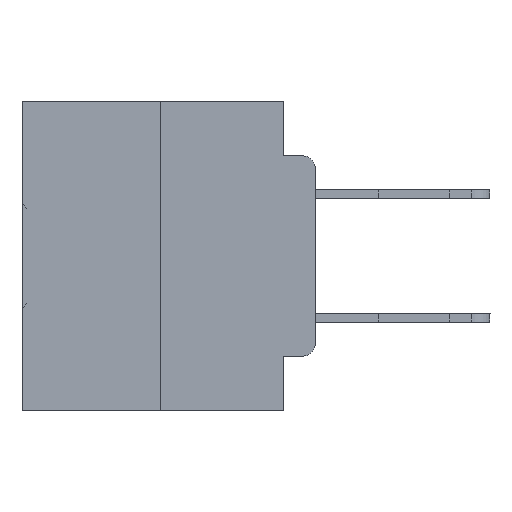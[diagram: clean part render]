
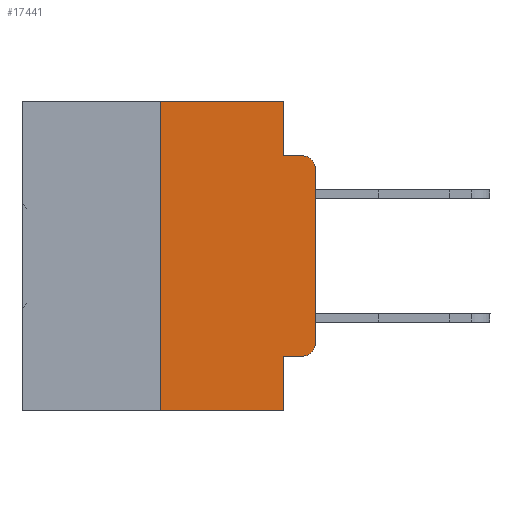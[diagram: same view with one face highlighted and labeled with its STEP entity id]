
A CAD part, left-side view. The second image highlights one B-rep face of the part: STEP entity #17441.
In plain terms, the highlighted planar face has unit normal (-1, 0, 0).
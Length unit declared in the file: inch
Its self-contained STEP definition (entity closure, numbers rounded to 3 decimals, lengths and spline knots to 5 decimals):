
#328 = VECTOR ( 'NONE', #32513, 39.37008 ) ;
#604 = EDGE_CURVE ( 'NONE', #28503, #11090, #23634, .T. ) ;
#620 = ORIENTED_EDGE ( 'NONE', *, *, #7553, .T. ) ;
#666 = CARTESIAN_POINT ( 'NONE',  ( 0., 0.02, -0.0885 ) ) ;
#913 = DIRECTION ( 'NONE',  ( 0., -1., 0. ) ) ;
#926 = CARTESIAN_POINT ( 'NONE',  ( 0., 0.051, -0.0885 ) ) ;
#1120 = EDGE_CURVE ( 'NONE', #25162, #10186, #12783, .T. ) ;
#1220 = DIRECTION ( 'NONE',  ( 0., 0., -1. ) ) ;
#1503 = AXIS2_PLACEMENT_3D ( 'NONE', #24187, #26630, #21522 ) ;
#1647 = DIRECTION ( 'NONE',  ( 0., 0., -1. ) ) ;
#1750 = CARTESIAN_POINT ( 'NONE',  ( 0., 0.25, -0.5 ) ) ;
#1977 = LINE ( 'NONE', #24766, #22276 ) ;
#2507 = DIRECTION ( 'NONE',  ( 0., 0., 1. ) ) ;
#3625 = DIRECTION ( 'NONE',  ( 0., 0., -1. ) ) ;
#4044 = CARTESIAN_POINT ( 'NONE',  ( 0., 0.051, -0.0885 ) ) ;
#5214 = VERTEX_POINT ( 'NONE', #25886 ) ;
#5692 = LINE ( 'NONE', #13133, #20597 ) ;
#6142 = VERTEX_POINT ( 'NONE', #18180 ) ;
#7553 = EDGE_CURVE ( 'NONE', #28503, #25162, #12108, .T. ) ;
#7687 = CARTESIAN_POINT ( 'NONE',  ( 0., 0.051, 0. ) ) ;
#8084 = ORIENTED_EDGE ( 'NONE', *, *, #31767, .T. ) ;
#8592 = ORIENTED_EDGE ( 'NONE', *, *, #604, .F. ) ;
#9708 = ORIENTED_EDGE ( 'NONE', *, *, #27085, .F. ) ;
#9734 = CARTESIAN_POINT ( 'NONE',  ( 0., 0.02, -0.3915 ) ) ;
#10186 = VERTEX_POINT ( 'NONE', #22478 ) ;
#10661 = EDGE_CURVE ( 'NONE', #28291, #11090, #28951, .T. ) ;
#10670 = LINE ( 'NONE', #926, #328 ) ;
#11090 = VERTEX_POINT ( 'NONE', #18429 ) ;
#11204 = CARTESIAN_POINT ( 'NONE',  ( 0., 0.051, -0.4115 ) ) ;
#12108 = LINE ( 'NONE', #24757, #22501 ) ;
#12713 = DIRECTION ( 'NONE',  ( 0., -1., 0. ) ) ;
#12783 = CIRCLE ( 'NONE', #13055, 0.02 ) ;
#12868 = DIRECTION ( 'NONE',  ( 0., 0., -1. ) ) ;
#13055 = AXIS2_PLACEMENT_3D ( 'NONE', #9734, #33575, #1647 ) ;
#13133 = CARTESIAN_POINT ( 'NONE',  ( 0., 0., 0. ) ) ;
#13678 = VECTOR ( 'NONE', #12868, 39.37008 ) ;
#13772 = EDGE_CURVE ( 'NONE', #29614, #30503, #14657, .T. ) ;
#13831 = ORIENTED_EDGE ( 'NONE', *, *, #27044, .F. ) ;
#14417 = VECTOR ( 'NONE', #12713, 39.37008 ) ;
#14657 = LINE ( 'NONE', #24811, #29194 ) ;
#14684 = DIRECTION ( 'NONE',  ( 0., -1., 0. ) ) ;
#15313 = CARTESIAN_POINT ( 'NONE',  ( 0., 0.25, 0. ) ) ;
#16434 = EDGE_CURVE ( 'NONE', #5214, #17668, #28692, .T. ) ;
#16657 = EDGE_CURVE ( 'NONE', #28291, #6142, #30323, .T. ) ;
#17441 = ADVANCED_FACE ( 'NONE', ( #17785 ), #19046, .F. ) ;
#17668 = VERTEX_POINT ( 'NONE', #666 ) ;
#17785 = FACE_OUTER_BOUND ( 'NONE', #25839, .T. ) ;
#18180 = CARTESIAN_POINT ( 'NONE',  ( 0., 0.25, 0. ) ) ;
#18429 = CARTESIAN_POINT ( 'NONE',  ( 0., 0.051, -0.5 ) ) ;
#19046 = PLANE ( 'NONE',  #1503 ) ;
#19600 = CARTESIAN_POINT ( 'NONE',  ( 0., 0.02, -0.1085 ) ) ;
#20140 = CARTESIAN_POINT ( 'NONE',  ( 0., 0.02, -0.4115 ) ) ;
#20597 = VECTOR ( 'NONE', #2507, 39.37008 ) ;
#20775 = ORIENTED_EDGE ( 'NONE', *, *, #16657, .F. ) ;
#20986 = DIRECTION ( 'NONE',  ( 0., 0., 1. ) ) ;
#21522 = DIRECTION ( 'NONE',  ( 0., 0., -1. ) ) ;
#22276 = VECTOR ( 'NONE', #14684, 39.37008 ) ;
#22478 = CARTESIAN_POINT ( 'NONE',  ( 0., 0., -0.3915 ) ) ;
#22501 = VECTOR ( 'NONE', #913, 39.37008 ) ;
#23634 = LINE ( 'NONE', #7687, #13678 ) ;
#24026 = ORIENTED_EDGE ( 'NONE', *, *, #10661, .T. ) ;
#24187 = CARTESIAN_POINT ( 'NONE',  ( 0., 0.473, 0. ) ) ;
#24757 = CARTESIAN_POINT ( 'NONE',  ( 0., 0.051, -0.4115 ) ) ;
#24766 = CARTESIAN_POINT ( 'NONE',  ( 0., 0.473, 0. ) ) ;
#24811 = CARTESIAN_POINT ( 'NONE',  ( 0., 0.051, 0. ) ) ;
#25162 = VERTEX_POINT ( 'NONE', #20140 ) ;
#25839 = EDGE_LOOP ( 'NONE', ( #8084, #26881, #13831, #30063, #9708, #20775, #24026, #8592, #620, #26279 ) ) ;
#25886 = CARTESIAN_POINT ( 'NONE',  ( 0., 0., -0.1085 ) ) ;
#26279 = ORIENTED_EDGE ( 'NONE', *, *, #1120, .T. ) ;
#26630 = DIRECTION ( 'NONE',  ( 1., 0., 0. ) ) ;
#26881 = ORIENTED_EDGE ( 'NONE', *, *, #16434, .T. ) ;
#27044 = EDGE_CURVE ( 'NONE', #30503, #17668, #10670, .T. ) ;
#27085 = EDGE_CURVE ( 'NONE', #6142, #29614, #1977, .T. ) ;
#27847 = DIRECTION ( 'NONE',  ( -1., 0., 0. ) ) ;
#28291 = VERTEX_POINT ( 'NONE', #1750 ) ;
#28503 = VERTEX_POINT ( 'NONE', #11204 ) ;
#28628 = CARTESIAN_POINT ( 'NONE',  ( 0., 0.473, -0.5 ) ) ;
#28692 = CIRCLE ( 'NONE', #31872, 0.02 ) ;
#28951 = LINE ( 'NONE', #28628, #14417 ) ;
#29104 = CARTESIAN_POINT ( 'NONE',  ( 0., 0.051, 0. ) ) ;
#29194 = VECTOR ( 'NONE', #3625, 39.37008 ) ;
#29614 = VERTEX_POINT ( 'NONE', #29104 ) ;
#30063 = ORIENTED_EDGE ( 'NONE', *, *, #13772, .F. ) ;
#30323 = LINE ( 'NONE', #15313, #30758 ) ;
#30503 = VERTEX_POINT ( 'NONE', #4044 ) ;
#30758 = VECTOR ( 'NONE', #20986, 39.37008 ) ;
#31767 = EDGE_CURVE ( 'NONE', #10186, #5214, #5692, .T. ) ;
#31872 = AXIS2_PLACEMENT_3D ( 'NONE', #19600, #27847, #1220 ) ;
#32513 = DIRECTION ( 'NONE',  ( 0., -1., 0. ) ) ;
#33575 = DIRECTION ( 'NONE',  ( -1., 0., 0. ) ) ;
